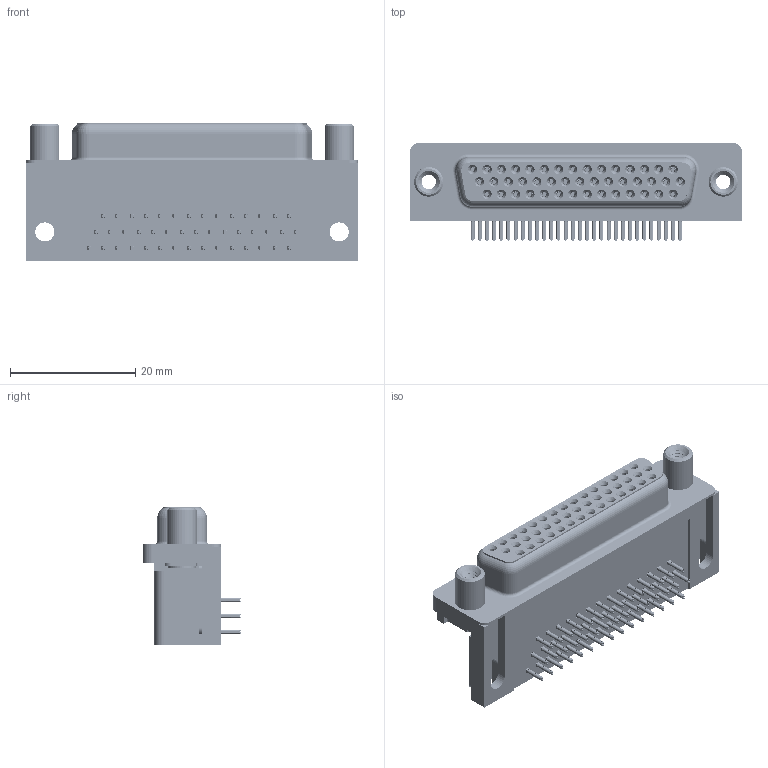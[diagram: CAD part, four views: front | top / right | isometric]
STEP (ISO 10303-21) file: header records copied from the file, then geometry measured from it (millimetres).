
FILE_DESCRIPTION (( 'STEP AP203' ), '1' );
FILE_NAME ('634-044-663-510.STEP', '2018-08-18T06:55:33', ( '' ), ( '' ), 'SwSTEP 2.0', 'SolidWorks 2016', '' );
FILE_SCHEMA (( 'CONFIG_CONTROL_DESIGN' ));
Length unit declared in the file: millimetre
Products named in the file (8): 634 Shell_44 Socket; Contact Bottom; Contact Middle; Contact Top; Thru Hole Board Mount; Round Threaded Standoff; 634-044-663-510; 634 Housing_44 Socket
Assembly tree (50 placements, depth 2):
  634-044-663-510
    634 Housing_44 Socket
    634 Shell_44 Socket
    Contact Bottom  x14
    Contact Middle  x15
    Contact Top  x15
    Thru Hole Board Mount  x2
    Round Threaded Standoff  x2
Bounding box: 53.04 x 15.73 x 22.1 mm (x, y, z)
Volume: 9445.2 mm3; surface area: 13466.4 mm2
Topology: 50 solids, 50 shells, 6529 faces, 17180 edges, 10786 vertices
Faces by surface type: plane 2919, bspline 1544, cylinder 1504, cone 540, torus 22
Entity records: 44852 total; most frequent: CARTESIAN_POINT 13736, ORIENTED_EDGE 6178, DIRECTION 5627, EDGE_CURVE 3089, VECTOR 2073, LINE 2073, VERTEX_POINT 1976, AXIS2_PLACEMENT_3D 1777
